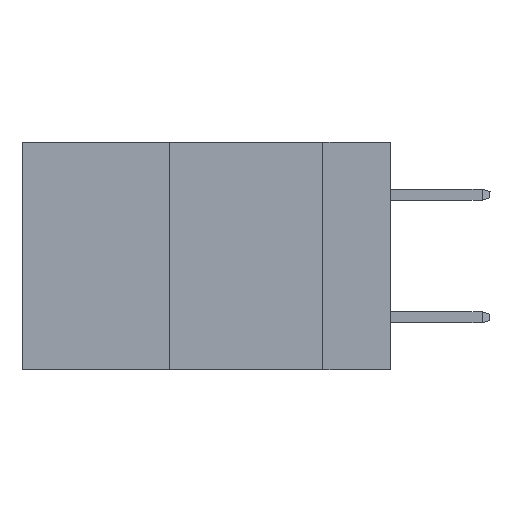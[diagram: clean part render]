
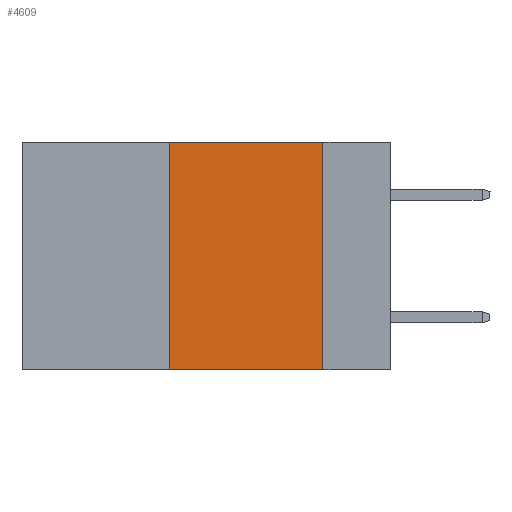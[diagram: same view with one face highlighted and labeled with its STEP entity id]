
A CAD part, left-side view. The second image highlights one B-rep face of the part: STEP entity #4609.
In plain terms, the highlighted planar face has unit normal (-1, 0, 0).
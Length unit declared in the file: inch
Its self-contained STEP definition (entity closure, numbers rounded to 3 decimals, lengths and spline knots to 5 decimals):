
#477 = ORIENTED_EDGE ( 'NONE', *, *, #7203, .F. ) ;
#799 = DIRECTION ( 'NONE',  ( 0., 0., 1. ) ) ;
#1220 = EDGE_CURVE ( 'NONE', #3096, #8737, #1360, .T. ) ;
#1360 = LINE ( 'NONE', #6307, #8862 ) ;
#1640 = ORIENTED_EDGE ( 'NONE', *, *, #8651, .F. ) ;
#1751 = VECTOR ( 'NONE', #2178, 39.37008 ) ;
#1828 = PLANE ( 'NONE',  #3610 ) ;
#2037 = DIRECTION ( 'NONE',  ( 1., 0., 0. ) ) ;
#2178 = DIRECTION ( 'NONE',  ( 0., 0., -1. ) ) ;
#3096 = VERTEX_POINT ( 'NONE', #5806 ) ;
#3610 = AXIS2_PLACEMENT_3D ( 'NONE', #9556, #2037, #3631 ) ;
#3631 = DIRECTION ( 'NONE',  ( 0., 0., -1. ) ) ;
#3774 = EDGE_LOOP ( 'NONE', ( #1640, #10123, #477, #10566 ) ) ;
#3991 = CARTESIAN_POINT ( 'NONE',  ( 0., 0.11, 0. ) ) ;
#4101 = LINE ( 'NONE', #3991, #1751 ) ;
#4609 = ADVANCED_FACE ( 'NONE', ( #9351 ), #1828, .F. ) ;
#4806 = DIRECTION ( 'NONE',  ( 0., -1., 0. ) ) ;
#4966 = LINE ( 'NONE', #8324, #7693 ) ;
#5806 = CARTESIAN_POINT ( 'NONE',  ( 0., 0.36, -0.37 ) ) ;
#6307 = CARTESIAN_POINT ( 'NONE',  ( 0., 0.6, -0.37 ) ) ;
#6967 = EDGE_CURVE ( 'NONE', #8967, #8595, #7231, .T. ) ;
#7021 = CARTESIAN_POINT ( 'NONE',  ( 0., 0.11, 0. ) ) ;
#7203 = EDGE_CURVE ( 'NONE', #3096, #8967, #4966, .T. ) ;
#7231 = LINE ( 'NONE', #9800, #7868 ) ;
#7693 = VECTOR ( 'NONE', #799, 39.37008 ) ;
#7868 = VECTOR ( 'NONE', #4806, 39.37008 ) ;
#8324 = CARTESIAN_POINT ( 'NONE',  ( 0., 0.36, 0. ) ) ;
#8595 = VERTEX_POINT ( 'NONE', #7021 ) ;
#8651 = EDGE_CURVE ( 'NONE', #8595, #8737, #4101, .T. ) ;
#8737 = VERTEX_POINT ( 'NONE', #9916 ) ;
#8862 = VECTOR ( 'NONE', #9704, 39.37008 ) ;
#8967 = VERTEX_POINT ( 'NONE', #9428 ) ;
#9351 = FACE_OUTER_BOUND ( 'NONE', #3774, .T. ) ;
#9428 = CARTESIAN_POINT ( 'NONE',  ( 0., 0.36, 0. ) ) ;
#9556 = CARTESIAN_POINT ( 'NONE',  ( 0., 0.6, 0. ) ) ;
#9704 = DIRECTION ( 'NONE',  ( 0., -1., 0. ) ) ;
#9800 = CARTESIAN_POINT ( 'NONE',  ( 0., 0.6, 0. ) ) ;
#9916 = CARTESIAN_POINT ( 'NONE',  ( 0., 0.11, -0.37 ) ) ;
#10123 = ORIENTED_EDGE ( 'NONE', *, *, #6967, .F. ) ;
#10566 = ORIENTED_EDGE ( 'NONE', *, *, #1220, .T. ) ;
